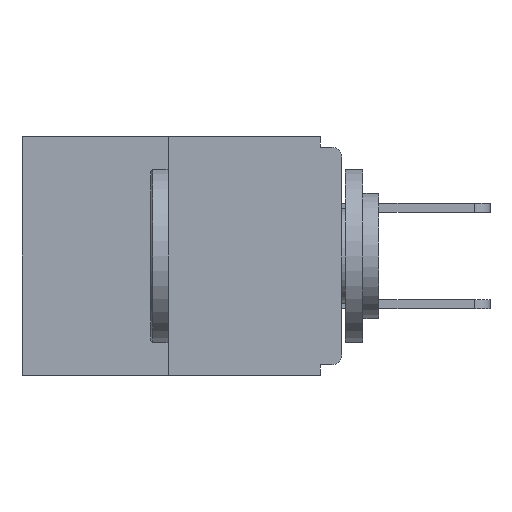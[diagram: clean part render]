
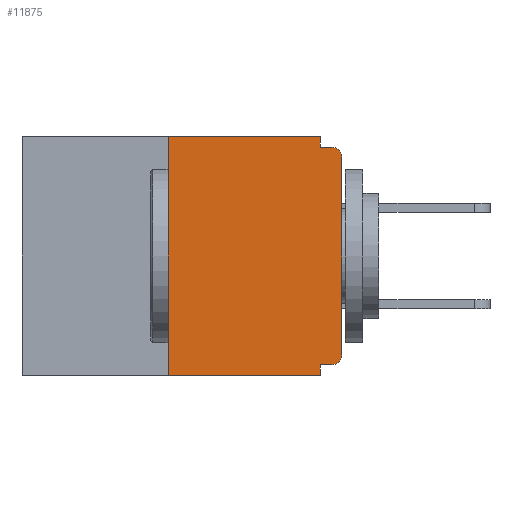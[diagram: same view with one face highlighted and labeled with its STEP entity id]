
A CAD part, left-side view. The second image highlights one B-rep face of the part: STEP entity #11875.
In plain terms, the highlighted planar face has unit normal (-1, 0, 0).
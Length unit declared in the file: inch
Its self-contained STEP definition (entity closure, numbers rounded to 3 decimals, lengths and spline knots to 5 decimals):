
#13 = DIRECTION ( 'NONE',  ( 0., 0., -1. ) ) ;
#25 = EDGE_CURVE ( 'NONE', #18632, #20489, #817, .T. ) ;
#817 = LINE ( 'NONE', #17268, #17096 ) ;
#1289 = EDGE_CURVE ( 'NONE', #20314, #4773, #6872, .T. ) ;
#1951 = DIRECTION ( 'NONE',  ( 0., -1., 0. ) ) ;
#3687 = VECTOR ( 'NONE', #30465, 39.37008 ) ;
#4332 = CARTESIAN_POINT ( 'NONE',  ( 0., 0., -0.313 ) ) ;
#4773 = VERTEX_POINT ( 'NONE', #4332 ) ;
#4885 = CARTESIAN_POINT ( 'NONE',  ( 0., 0.031, 0. ) ) ;
#5215 = CARTESIAN_POINT ( 'NONE',  ( 0., 0.015, -0.015 ) ) ;
#5383 = ORIENTED_EDGE ( 'NONE', *, *, #29170, .T. ) ;
#5487 = VERTEX_POINT ( 'NONE', #5215 ) ;
#5654 = EDGE_CURVE ( 'NONE', #20314, #29908, #19541, .T. ) ;
#5739 = CARTESIAN_POINT ( 'NONE',  ( 0., 0., -0.328 ) ) ;
#5928 = CARTESIAN_POINT ( 'NONE',  ( 0., 0.25, -0.343 ) ) ;
#6529 = VERTEX_POINT ( 'NONE', #9209 ) ;
#6554 = ORIENTED_EDGE ( 'NONE', *, *, #31038, .F. ) ;
#6594 = FACE_OUTER_BOUND ( 'NONE', #22238, .T. ) ;
#6680 = PLANE ( 'NONE',  #22768 ) ;
#6872 = CIRCLE ( 'NONE', #17240, 0.015 ) ;
#7044 = DIRECTION ( 'NONE',  ( 0., -1., 0. ) ) ;
#7804 = ORIENTED_EDGE ( 'NONE', *, *, #5654, .F. ) ;
#8081 = CARTESIAN_POINT ( 'NONE',  ( 0., 0.015, -0.328 ) ) ;
#8935 = LINE ( 'NONE', #4885, #20126 ) ;
#8962 = LINE ( 'NONE', #9790, #22852 ) ;
#9058 = CARTESIAN_POINT ( 'NONE',  ( 0., 0.25, 0. ) ) ;
#9209 = CARTESIAN_POINT ( 'NONE',  ( 0., 0., -0.03 ) ) ;
#9267 = VECTOR ( 'NONE', #16905, 39.37008 ) ;
#9306 = VECTOR ( 'NONE', #17843, 39.37008 ) ;
#9790 = CARTESIAN_POINT ( 'NONE',  ( 0., 0.46, -0.343 ) ) ;
#9822 = ORIENTED_EDGE ( 'NONE', *, *, #12240, .F. ) ;
#11254 = DIRECTION ( 'NONE',  ( -1., 0., 0. ) ) ;
#11558 = ORIENTED_EDGE ( 'NONE', *, *, #1289, .T. ) ;
#11717 = DIRECTION ( 'NONE',  ( 0., 0., -1. ) ) ;
#11875 = ADVANCED_FACE ( 'NONE', ( #6594 ), #6680, .F. ) ;
#12234 = VERTEX_POINT ( 'NONE', #5928 ) ;
#12240 = EDGE_CURVE ( 'NONE', #12234, #18632, #16292, .T. ) ;
#12401 = DIRECTION ( 'NONE',  ( 0., 0., 1. ) ) ;
#14269 = CARTESIAN_POINT ( 'NONE',  ( 0., 0., -0.015 ) ) ;
#14425 = EDGE_CURVE ( 'NONE', #4773, #6529, #27677, .T. ) ;
#16292 = LINE ( 'NONE', #18281, #9306 ) ;
#16360 = ORIENTED_EDGE ( 'NONE', *, *, #20863, .F. ) ;
#16905 = DIRECTION ( 'NONE',  ( 0., 0., -1. ) ) ;
#17096 = VECTOR ( 'NONE', #31590, 39.37008 ) ;
#17240 = AXIS2_PLACEMENT_3D ( 'NONE', #18312, #30676, #30790 ) ;
#17268 = CARTESIAN_POINT ( 'NONE',  ( 0., 0.46, 0. ) ) ;
#17843 = DIRECTION ( 'NONE',  ( 0., 0., 1. ) ) ;
#18281 = CARTESIAN_POINT ( 'NONE',  ( 0., 0.25, 0. ) ) ;
#18312 = CARTESIAN_POINT ( 'NONE',  ( 0., 0.015, -0.313 ) ) ;
#18356 = VERTEX_POINT ( 'NONE', #18513 ) ;
#18379 = CARTESIAN_POINT ( 'NONE',  ( 0., 0.031, 0. ) ) ;
#18513 = CARTESIAN_POINT ( 'NONE',  ( 0., 0.031, -0.015 ) ) ;
#18632 = VERTEX_POINT ( 'NONE', #9058 ) ;
#19301 = LINE ( 'NONE', #22246, #9267 ) ;
#19541 = LINE ( 'NONE', #5739, #3687 ) ;
#20126 = VECTOR ( 'NONE', #13, 39.37008 ) ;
#20314 = VERTEX_POINT ( 'NONE', #8081 ) ;
#20489 = VERTEX_POINT ( 'NONE', #18379 ) ;
#20695 = CARTESIAN_POINT ( 'NONE',  ( 0., 0.031, -0.328 ) ) ;
#20724 = ORIENTED_EDGE ( 'NONE', *, *, #23983, .T. ) ;
#20863 = EDGE_CURVE ( 'NONE', #29908, #27491, #19301, .T. ) ;
#20956 = CARTESIAN_POINT ( 'NONE',  ( 0., 0.015, -0.03 ) ) ;
#21449 = CIRCLE ( 'NONE', #27926, 0.015 ) ;
#22238 = EDGE_LOOP ( 'NONE', ( #26799, #9822, #5383, #16360, #7804, #11558, #32012, #20724, #6554, #30026 ) ) ;
#22246 = CARTESIAN_POINT ( 'NONE',  ( 0., 0.031, -0.343 ) ) ;
#22301 = CARTESIAN_POINT ( 'NONE',  ( 0., 0., 0. ) ) ;
#22768 = AXIS2_PLACEMENT_3D ( 'NONE', #28733, #28627, #11717 ) ;
#22852 = VECTOR ( 'NONE', #7044, 39.37008 ) ;
#23983 = EDGE_CURVE ( 'NONE', #6529, #5487, #21449, .T. ) ;
#26799 = ORIENTED_EDGE ( 'NONE', *, *, #25, .F. ) ;
#27491 = VERTEX_POINT ( 'NONE', #30098 ) ;
#27677 = LINE ( 'NONE', #22301, #31548 ) ;
#27926 = AXIS2_PLACEMENT_3D ( 'NONE', #20956, #11254, #30965 ) ;
#28627 = DIRECTION ( 'NONE',  ( 1., 0., 0. ) ) ;
#28733 = CARTESIAN_POINT ( 'NONE',  ( 0., 0.46, 0. ) ) ;
#28922 = VECTOR ( 'NONE', #1951, 39.37008 ) ;
#29170 = EDGE_CURVE ( 'NONE', #12234, #27491, #8962, .T. ) ;
#29275 = EDGE_CURVE ( 'NONE', #20489, #18356, #8935, .T. ) ;
#29908 = VERTEX_POINT ( 'NONE', #20695 ) ;
#30026 = ORIENTED_EDGE ( 'NONE', *, *, #29275, .F. ) ;
#30098 = CARTESIAN_POINT ( 'NONE',  ( 0., 0.031, -0.343 ) ) ;
#30465 = DIRECTION ( 'NONE',  ( 0., 1., 0. ) ) ;
#30466 = LINE ( 'NONE', #14269, #28922 ) ;
#30676 = DIRECTION ( 'NONE',  ( -1., 0., 0. ) ) ;
#30790 = DIRECTION ( 'NONE',  ( 0., 0., -1. ) ) ;
#30965 = DIRECTION ( 'NONE',  ( 0., 0., -1. ) ) ;
#31038 = EDGE_CURVE ( 'NONE', #18356, #5487, #30466, .T. ) ;
#31548 = VECTOR ( 'NONE', #12401, 39.37008 ) ;
#31590 = DIRECTION ( 'NONE',  ( 0., -1., 0. ) ) ;
#32012 = ORIENTED_EDGE ( 'NONE', *, *, #14425, .T. ) ;
